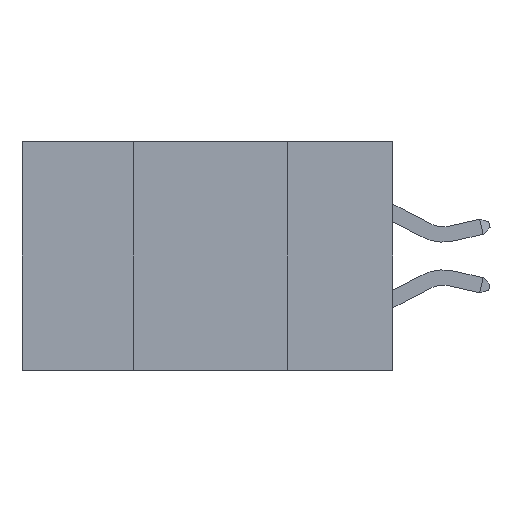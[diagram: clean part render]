
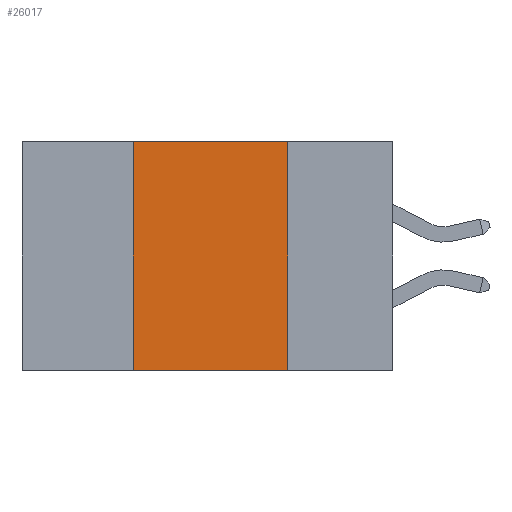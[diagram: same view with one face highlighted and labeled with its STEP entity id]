
A CAD part, left-side view. The second image highlights one B-rep face of the part: STEP entity #26017.
In plain terms, the highlighted planar face has unit normal (-1, 0, 0).
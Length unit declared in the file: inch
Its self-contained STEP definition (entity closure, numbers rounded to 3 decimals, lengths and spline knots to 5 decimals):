
#1367 = VERTEX_POINT ( 'NONE', #15555 ) ;
#3278 = VECTOR ( 'NONE', #22905, 39.37008 ) ;
#4872 = CARTESIAN_POINT ( 'NONE',  ( 0., 0.42, 0. ) ) ;
#5158 = DIRECTION ( 'NONE',  ( 0., -1., 0. ) ) ;
#5347 = CARTESIAN_POINT ( 'NONE',  ( 0., 0.6, -0.37 ) ) ;
#5574 = VERTEX_POINT ( 'NONE', #16129 ) ;
#11529 = CARTESIAN_POINT ( 'NONE',  ( 0., 0.6, 0. ) ) ;
#12267 = LINE ( 'NONE', #15205, #17361 ) ;
#13025 = FACE_OUTER_BOUND ( 'NONE', #15365, .T. ) ;
#13581 = DIRECTION ( 'NONE',  ( 0., 0., -1. ) ) ;
#14085 = VERTEX_POINT ( 'NONE', #25830 ) ;
#14827 = LINE ( 'NONE', #11529, #3278 ) ;
#15164 = AXIS2_PLACEMENT_3D ( 'NONE', #24953, #27732, #13581 ) ;
#15205 = CARTESIAN_POINT ( 'NONE',  ( 0., 0.17, 0. ) ) ;
#15365 = EDGE_LOOP ( 'NONE', ( #15600, #31637, #34705, #24096 ) ) ;
#15555 = CARTESIAN_POINT ( 'NONE',  ( 0., 0.17, -0.37 ) ) ;
#15600 = ORIENTED_EDGE ( 'NONE', *, *, #23324, .F. ) ;
#16129 = CARTESIAN_POINT ( 'NONE',  ( 0., 0.42, 0. ) ) ;
#17164 = EDGE_CURVE ( 'NONE', #5574, #14085, #14827, .T. ) ;
#17361 = VECTOR ( 'NONE', #34842, 39.37008 ) ;
#17574 = VECTOR ( 'NONE', #5158, 39.37008 ) ;
#19082 = PLANE ( 'NONE',  #15164 ) ;
#20664 = VERTEX_POINT ( 'NONE', #35359 ) ;
#22905 = DIRECTION ( 'NONE',  ( 0., -1., 0. ) ) ;
#23324 = EDGE_CURVE ( 'NONE', #14085, #1367, #12267, .T. ) ;
#24096 = ORIENTED_EDGE ( 'NONE', *, *, #26722, .T. ) ;
#24953 = CARTESIAN_POINT ( 'NONE',  ( 0., 0.6, 0. ) ) ;
#25031 = LINE ( 'NONE', #5347, #17574 ) ;
#25830 = CARTESIAN_POINT ( 'NONE',  ( 0., 0.17, 0. ) ) ;
#26017 = ADVANCED_FACE ( 'NONE', ( #13025 ), #19082, .F. ) ;
#26722 = EDGE_CURVE ( 'NONE', #20664, #1367, #25031, .T. ) ;
#27704 = LINE ( 'NONE', #4872, #35859 ) ;
#27732 = DIRECTION ( 'NONE',  ( 1., 0., 0. ) ) ;
#31102 = EDGE_CURVE ( 'NONE', #20664, #5574, #27704, .T. ) ;
#31637 = ORIENTED_EDGE ( 'NONE', *, *, #17164, .F. ) ;
#34705 = ORIENTED_EDGE ( 'NONE', *, *, #31102, .F. ) ;
#34842 = DIRECTION ( 'NONE',  ( 0., 0., -1. ) ) ;
#35359 = CARTESIAN_POINT ( 'NONE',  ( 0., 0.42, -0.37 ) ) ;
#35859 = VECTOR ( 'NONE', #35945, 39.37008 ) ;
#35945 = DIRECTION ( 'NONE',  ( 0., 0., 1. ) ) ;
